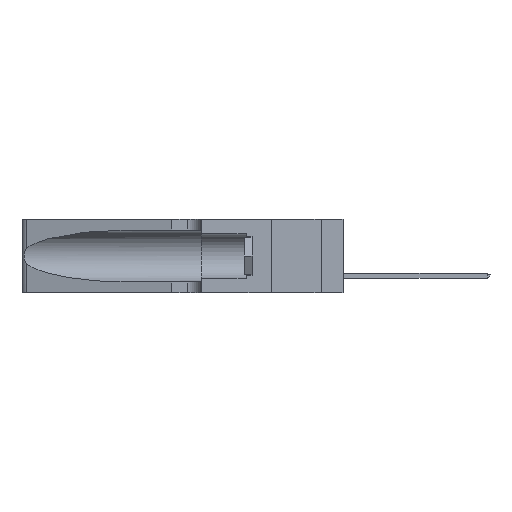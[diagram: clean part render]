
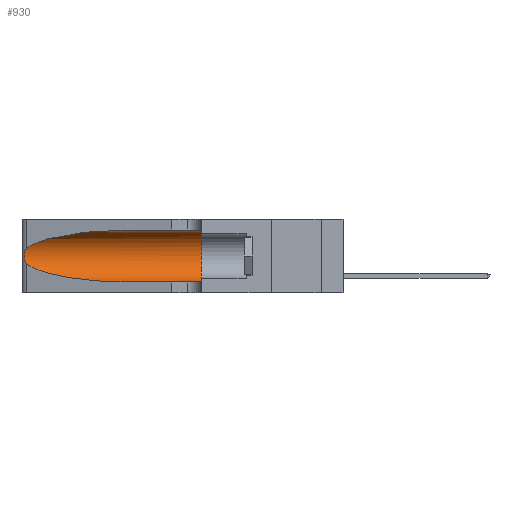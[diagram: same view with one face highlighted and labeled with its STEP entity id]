
A CAD part, left-side view. The second image highlights one B-rep face of the part: STEP entity #930.
In plain terms, the highlighted cylindrical face has radius 3.308 mm (diameter 6.617 mm), a partial arc.
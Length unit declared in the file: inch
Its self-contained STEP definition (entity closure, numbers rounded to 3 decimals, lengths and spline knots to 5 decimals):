
#269 = DIRECTION ( 'NONE',  ( 0., -1., 0. ) ) ;
#528 = EDGE_CURVE ( 'NONE', #23491, #2638, #8796, .T. ) ;
#604 = CARTESIAN_POINT ( 'NONE',  ( 0.1305, 0.72297, 0.31525 ) ) ;
#930 = ADVANCED_FACE ( 'NONE', ( #4669 ), #10574, .F. ) ;
#933 = CARTESIAN_POINT ( 'NONE',  ( 0.25487, 1.22718, 0.22369 ) ) ;
#2281 = ORIENTED_EDGE ( 'NONE', *, *, #528, .T. ) ;
#2638 = VERTEX_POINT ( 'NONE', #12844 ) ;
#2722 = ORIENTED_EDGE ( 'NONE', *, *, #24066, .T. ) ;
#2744 = CARTESIAN_POINT ( 'NONE',  ( 0.18966, 0.96281, 0.05475 ) ) ;
#3214 = CARTESIAN_POINT ( 'NONE',  ( 0.26075, 1.23896, 0.178 ) ) ;
#4669 = FACE_OUTER_BOUND ( 'NONE', #5663, .T. ) ;
#4879 = VECTOR ( 'NONE', #13916, 39.37008 ) ;
#5663 = EDGE_LOOP ( 'NONE', ( #18513, #2281, #2722, #25790, #17494, #9356 ) ) ;
#6797 = CIRCLE ( 'NONE', #16350, 0.13025 ) ;
#7258 = CARTESIAN_POINT ( 'NONE',  ( 0.26018, 1.23835, 0.19895 ) ) ;
#7608 = VECTOR ( 'NONE', #269, 39.37008 ) ;
#7674 = VERTEX_POINT ( 'NONE', #11588 ) ;
#8796 = B_SPLINE_CURVE_WITH_KNOTS ( 'NONE', 3,
 ( #933, #15573, #21438, #15856, #13653, #7258, #23993, #3214, #13750, #9450, #24273, #17773, #17860, #15758 ),
 .UNSPECIFIED., .F., .F.,
 ( 4, 2, 2, 2, 2, 2, 4 ),
 ( 0., 0.00027, 0.00053, 0.00107, 0.0016, 0.00187, 0.00214 ),
 .UNSPECIFIED. ) ;
#8923 = EDGE_CURVE ( 'NONE', #12123, #14605, #6797, .T. ) ;
#9356 = ORIENTED_EDGE ( 'NONE', *, *, #11937, .F. ) ;
#9450 = CARTESIAN_POINT ( 'NONE',  ( 0.25856, 1.23593, 0.16098 ) ) ;
#10212 = CARTESIAN_POINT ( 'NONE',  ( 0.25487, 1.22718, 0.22369 ) ) ;
#10574 = CYLINDRICAL_SURFACE ( 'NONE', #15366, 0.13025 ) ;
#10641 = DIRECTION ( 'NONE',  ( 0., -1., 0. ) ) ;
#11462 = CARTESIAN_POINT ( 'NONE',  ( 0.18966, 0.96281, 0.31525 ) ) ;
#11551 = CARTESIAN_POINT ( 'NONE',  ( 0.25487, 1.22718, 0.22369 ) ) ;
#11588 = CARTESIAN_POINT ( 'NONE',  ( 0.1305, 0.72297, 0.05475 ) ) ;
#11724 = CARTESIAN_POINT ( 'NONE',  ( 0.1305, 1.61858, 0.05475 ) ) ;
#11937 = EDGE_CURVE ( 'NONE', #15740, #12123, #13814, .T. ) ;
#12123 = VERTEX_POINT ( 'NONE', #20726 ) ;
#12479 =( BOUNDED_CURVE ( )  B_SPLINE_CURVE ( 3, ( #19777, #11462, #24089, #11551 ),
 .UNSPECIFIED., .F., .F. ) 
 B_SPLINE_CURVE_WITH_KNOTS ( ( 4, 4 ),
 ( 1.5708, 2.84003 ),
 .UNSPECIFIED. ) 
 CURVE ( )  GEOMETRIC_REPRESENTATION_ITEM ( )  RATIONAL_B_SPLINE_CURVE ( ( 1., 0.87, 0.87, 1. ) ) 
 REPRESENTATION_ITEM ( '' )  );
#12844 = CARTESIAN_POINT ( 'NONE',  ( 0.25487, 1.22718, 0.14631 ) ) ;
#13168 = DIRECTION ( 'NONE',  ( 0., 1., 0. ) ) ;
#13345 = CARTESIAN_POINT ( 'NONE',  ( 0.1305, 0.72297, 0.05475 ) ) ;
#13653 = CARTESIAN_POINT ( 'NONE',  ( 0.25854, 1.2359, 0.20912 ) ) ;
#13750 = CARTESIAN_POINT ( 'NONE',  ( 0.26017, 1.23833, 0.17102 ) ) ;
#13814 = LINE ( 'NONE', #21133, #7608 ) ;
#13916 = DIRECTION ( 'NONE',  ( 0., -1., 0. ) ) ;
#14605 = VERTEX_POINT ( 'NONE', #17019 ) ;
#14954 = CARTESIAN_POINT ( 'NONE',  ( 0.1305, 1.61858, 0.185 ) ) ;
#15101 = CARTESIAN_POINT ( 'NONE',  ( 0.1305, 0.35, 0.185 ) ) ;
#15366 = AXIS2_PLACEMENT_3D ( 'NONE', #14954, #10641, #16870 ) ;
#15573 = CARTESIAN_POINT ( 'NONE',  ( 0.25555, 1.22994, 0.2215 ) ) ;
#15740 = VERTEX_POINT ( 'NONE', #604 ) ;
#15758 = CARTESIAN_POINT ( 'NONE',  ( 0.25487, 1.22718, 0.14631 ) ) ;
#15856 = CARTESIAN_POINT ( 'NONE',  ( 0.25787, 1.23484, 0.2124 ) ) ;
#16350 = AXIS2_PLACEMENT_3D ( 'NONE', #15101, #13168, #23498 ) ;
#16688 = EDGE_CURVE ( 'NONE', #7674, #14605, #23224, .T. ) ;
#16870 = DIRECTION ( 'NONE',  ( 0., 0., -1. ) ) ;
#17019 = CARTESIAN_POINT ( 'NONE',  ( 0.1305, 0.35, 0.05475 ) ) ;
#17304 =( BOUNDED_CURVE ( )  B_SPLINE_CURVE ( 3, ( #23785, #23509, #2744, #13345 ),
 .UNSPECIFIED., .F., .F. ) 
 B_SPLINE_CURVE_WITH_KNOTS ( ( 4, 4 ),
 ( 3.44316, 4.71239 ),
 .UNSPECIFIED. ) 
 CURVE ( )  GEOMETRIC_REPRESENTATION_ITEM ( )  RATIONAL_B_SPLINE_CURVE ( ( 1., 0.87, 0.87, 1. ) ) 
 REPRESENTATION_ITEM ( '' )  );
#17494 = ORIENTED_EDGE ( 'NONE', *, *, #8923, .F. ) ;
#17773 = CARTESIAN_POINT ( 'NONE',  ( 0.25639, 1.23186, 0.15144 ) ) ;
#17860 = CARTESIAN_POINT ( 'NONE',  ( 0.25555, 1.22993, 0.14849 ) ) ;
#18438 = EDGE_CURVE ( 'NONE', #15740, #23491, #12479, .T. ) ;
#18513 = ORIENTED_EDGE ( 'NONE', *, *, #18438, .T. ) ;
#19777 = CARTESIAN_POINT ( 'NONE',  ( 0.1305, 0.72297, 0.31525 ) ) ;
#20726 = CARTESIAN_POINT ( 'NONE',  ( 0.1305, 0.35, 0.31525 ) ) ;
#21133 = CARTESIAN_POINT ( 'NONE',  ( 0.1305, 1.61858, 0.31525 ) ) ;
#21438 = CARTESIAN_POINT ( 'NONE',  ( 0.25639, 1.23184, 0.21858 ) ) ;
#23224 = LINE ( 'NONE', #11724, #4879 ) ;
#23491 = VERTEX_POINT ( 'NONE', #10212 ) ;
#23498 = DIRECTION ( 'NONE',  ( 0., 0., 1. ) ) ;
#23509 = CARTESIAN_POINT ( 'NONE',  ( 0.2373, 1.15595, 0.08982 ) ) ;
#23785 = CARTESIAN_POINT ( 'NONE',  ( 0.25487, 1.22718, 0.14631 ) ) ;
#23993 = CARTESIAN_POINT ( 'NONE',  ( 0.26075, 1.23896, 0.19203 ) ) ;
#24066 = EDGE_CURVE ( 'NONE', #2638, #7674, #17304, .T. ) ;
#24089 = CARTESIAN_POINT ( 'NONE',  ( 0.2373, 1.15595, 0.28018 ) ) ;
#24273 = CARTESIAN_POINT ( 'NONE',  ( 0.25789, 1.23486, 0.15765 ) ) ;
#25790 = ORIENTED_EDGE ( 'NONE', *, *, #16688, .T. ) ;
